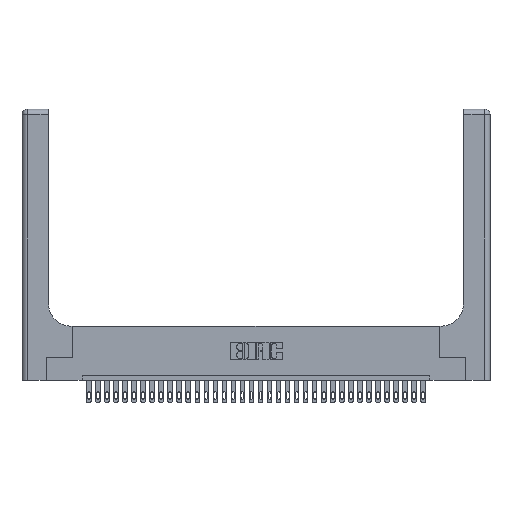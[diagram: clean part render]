
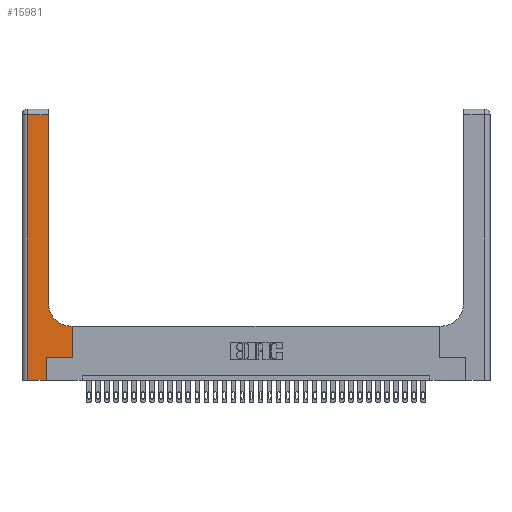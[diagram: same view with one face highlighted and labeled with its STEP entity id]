
A CAD part, top view. The second image highlights one B-rep face of the part: STEP entity #15981.
In plain terms, the highlighted planar face has unit normal (0, 0, 1).
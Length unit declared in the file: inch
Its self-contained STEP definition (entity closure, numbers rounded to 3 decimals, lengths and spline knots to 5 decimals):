
#297 = EDGE_CURVE ( 'NONE', #8570, #23124, #25053, .T. ) ;
#554 = ORIENTED_EDGE ( 'NONE', *, *, #30139, .T. ) ;
#796 = CARTESIAN_POINT ( 'NONE',  ( 0.2915, 0.85, 0.37 ) ) ;
#2382 = EDGE_CURVE ( 'NONE', #9921, #11789, #11618, .T. ) ;
#3059 = FACE_OUTER_BOUND ( 'NONE', #13101, .T. ) ;
#3462 = LINE ( 'NONE', #25270, #17103 ) ;
#3591 = LINE ( 'NONE', #25000, #13503 ) ;
#4837 = CARTESIAN_POINT ( 'NONE',  ( 0.06, 2.94, 0.37 ) ) ;
#5050 = LINE ( 'NONE', #22835, #13307 ) ;
#5078 = VERTEX_POINT ( 'NONE', #15640 ) ;
#5843 = CARTESIAN_POINT ( 'NONE',  ( 0., 0., 0.37 ) ) ;
#5997 = ORIENTED_EDGE ( 'NONE', *, *, #297, .T. ) ;
#6046 = EDGE_CURVE ( 'NONE', #21254, #7218, #6069, .T. ) ;
#6069 = LINE ( 'NONE', #24688, #13530 ) ;
#6249 = ORIENTED_EDGE ( 'NONE', *, *, #6046, .T. ) ;
#7218 = VERTEX_POINT ( 'NONE', #22046 ) ;
#7273 = VECTOR ( 'NONE', #30697, 39.37008 ) ;
#8149 = ORIENTED_EDGE ( 'NONE', *, *, #10806, .T. ) ;
#8452 = VERTEX_POINT ( 'NONE', #4837 ) ;
#8570 = VERTEX_POINT ( 'NONE', #29598 ) ;
#8813 = DIRECTION ( 'NONE',  ( 0., 0., -1. ) ) ;
#8960 = ORIENTED_EDGE ( 'NONE', *, *, #2382, .T. ) ;
#9056 = ORIENTED_EDGE ( 'NONE', *, *, #34193, .T. ) ;
#9619 = DIRECTION ( 'NONE',  ( 0., 1., 0. ) ) ;
#9909 = LINE ( 'NONE', #5843, #30164 ) ;
#9921 = VERTEX_POINT ( 'NONE', #23113 ) ;
#10298 = CARTESIAN_POINT ( 'NONE',  ( 0.2915, 2.94, 0.37 ) ) ;
#10477 = DIRECTION ( 'NONE',  ( 0., 0., -1. ) ) ;
#10806 = EDGE_CURVE ( 'NONE', #8452, #5078, #3462, .T. ) ;
#11618 = CIRCLE ( 'NONE', #16823, 0.25 ) ;
#11789 = VERTEX_POINT ( 'NONE', #796 ) ;
#12722 = EDGE_CURVE ( 'NONE', #11789, #26653, #5050, .T. ) ;
#13101 = EDGE_LOOP ( 'NONE', ( #28636, #16222, #8149, #15822, #5997, #9056, #6249, #554, #8960 ) ) ;
#13307 = VECTOR ( 'NONE', #9619, 39.37008 ) ;
#13503 = VECTOR ( 'NONE', #24667, 39.37008 ) ;
#13530 = VECTOR ( 'NONE', #24462, 39.37008 ) ;
#14186 = DIRECTION ( 'NONE',  ( 1., 0., 0. ) ) ;
#14660 = VECTOR ( 'NONE', #24583, 39.37008 ) ;
#15056 = DIRECTION ( 'NONE',  ( -1., 0., 0. ) ) ;
#15640 = CARTESIAN_POINT ( 'NONE',  ( 0.06, 0., 0.37 ) ) ;
#15822 = ORIENTED_EDGE ( 'NONE', *, *, #19492, .T. ) ;
#15981 = ADVANCED_FACE ( 'NONE', ( #3059 ), #19855, .F. ) ;
#16222 = ORIENTED_EDGE ( 'NONE', *, *, #18600, .T. ) ;
#16823 = AXIS2_PLACEMENT_3D ( 'NONE', #22039, #8813, #14186 ) ;
#17103 = VECTOR ( 'NONE', #25035, 39.37008 ) ;
#18600 = EDGE_CURVE ( 'NONE', #26653, #8452, #26425, .T. ) ;
#18980 = CARTESIAN_POINT ( 'NONE',  ( 0.269, 0.25, 0.37 ) ) ;
#19492 = EDGE_CURVE ( 'NONE', #5078, #8570, #9909, .T. ) ;
#19855 = PLANE ( 'NONE',  #21569 ) ;
#21254 = VERTEX_POINT ( 'NONE', #33098 ) ;
#21569 = AXIS2_PLACEMENT_3D ( 'NONE', #30476, #10477, #31546 ) ;
#21876 = VECTOR ( 'NONE', #15056, 39.37008 ) ;
#22039 = CARTESIAN_POINT ( 'NONE',  ( 0.5415, 0.85, 0.37 ) ) ;
#22046 = CARTESIAN_POINT ( 'NONE',  ( 0.5585, 0.6, 0.37 ) ) ;
#22835 = CARTESIAN_POINT ( 'NONE',  ( 0.2915, 3., 0.37 ) ) ;
#23113 = CARTESIAN_POINT ( 'NONE',  ( 0.5415, 0.6, 0.37 ) ) ;
#23124 = VERTEX_POINT ( 'NONE', #18980 ) ;
#24462 = DIRECTION ( 'NONE',  ( 0., 1., 0. ) ) ;
#24478 = DIRECTION ( 'NONE',  ( 1., 0., 0. ) ) ;
#24583 = DIRECTION ( 'NONE',  ( 1., 0., 0. ) ) ;
#24667 = DIRECTION ( 'NONE',  ( -1., 0., 0. ) ) ;
#24688 = CARTESIAN_POINT ( 'NONE',  ( 0.5585, 0.25, 0.37 ) ) ;
#24921 = CARTESIAN_POINT ( 'NONE',  ( 0.269, 0.25, 0.37 ) ) ;
#25000 = CARTESIAN_POINT ( 'NONE',  ( 0.2915, 0.6, 0.37 ) ) ;
#25035 = DIRECTION ( 'NONE',  ( 0., -1., 0. ) ) ;
#25053 = LINE ( 'NONE', #31052, #7273 ) ;
#25270 = CARTESIAN_POINT ( 'NONE',  ( 0.06, 3., 0.37 ) ) ;
#26425 = LINE ( 'NONE', #33567, #21876 ) ;
#26651 = LINE ( 'NONE', #24921, #14660 ) ;
#26653 = VERTEX_POINT ( 'NONE', #10298 ) ;
#28636 = ORIENTED_EDGE ( 'NONE', *, *, #12722, .T. ) ;
#29598 = CARTESIAN_POINT ( 'NONE',  ( 0.269, 0., 0.37 ) ) ;
#30139 = EDGE_CURVE ( 'NONE', #7218, #9921, #3591, .T. ) ;
#30164 = VECTOR ( 'NONE', #24478, 39.37008 ) ;
#30476 = CARTESIAN_POINT ( 'NONE',  ( 0., 3., 0.37 ) ) ;
#30697 = DIRECTION ( 'NONE',  ( 0., 1., 0. ) ) ;
#31052 = CARTESIAN_POINT ( 'NONE',  ( 0.269, 0., 0.37 ) ) ;
#31546 = DIRECTION ( 'NONE',  ( -1., 0., 0. ) ) ;
#33098 = CARTESIAN_POINT ( 'NONE',  ( 0.5585, 0.25, 0.37 ) ) ;
#33567 = CARTESIAN_POINT ( 'NONE',  ( 0., 2.94, 0.37 ) ) ;
#34193 = EDGE_CURVE ( 'NONE', #23124, #21254, #26651, .T. ) ;
